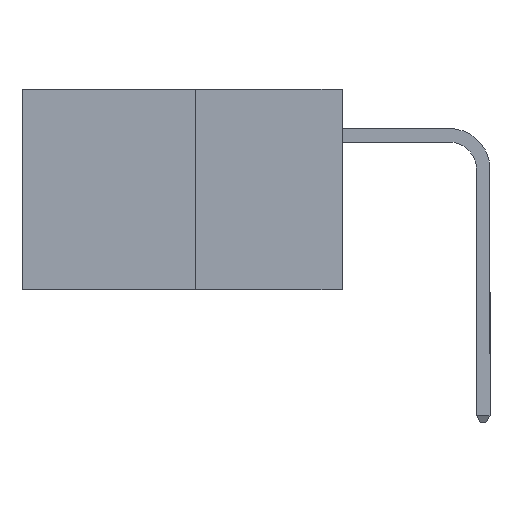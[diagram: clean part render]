
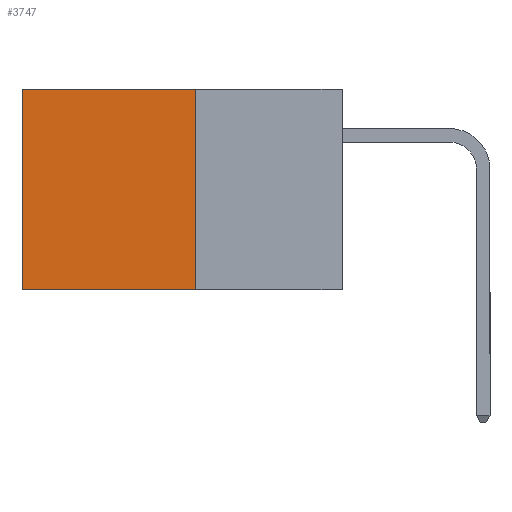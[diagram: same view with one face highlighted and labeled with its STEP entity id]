
A CAD part, left-side view. The second image highlights one B-rep face of the part: STEP entity #3747.
In plain terms, the highlighted planar face has unit normal (-1, 0, 0).
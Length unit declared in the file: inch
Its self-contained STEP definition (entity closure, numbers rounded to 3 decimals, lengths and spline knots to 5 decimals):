
#99 = LINE ( 'NONE', #5122, #6754 ) ;
#448 = DIRECTION ( 'NONE',  ( 0., 0., -1. ) ) ;
#484 = LINE ( 'NONE', #10018, #7142 ) ;
#1225 = ORIENTED_EDGE ( 'NONE', *, *, #4623, .T. ) ;
#1932 = CARTESIAN_POINT ( 'NONE',  ( 0.277, 0.27, -0.37 ) ) ;
#1987 = VECTOR ( 'NONE', #2751, 39.37008 ) ;
#2191 = FACE_OUTER_BOUND ( 'NONE', #2193, .T. ) ;
#2193 = EDGE_LOOP ( 'NONE', ( #1225, #6839, #4777, #4399 ) ) ;
#2557 = CARTESIAN_POINT ( 'NONE',  ( 0.277, 0.27, 0. ) ) ;
#2565 = CARTESIAN_POINT ( 'NONE',  ( 0.277, 0.27, 0. ) ) ;
#2669 = DIRECTION ( 'NONE',  ( 0., 0., -1. ) ) ;
#2751 = DIRECTION ( 'NONE',  ( 0., 1., 0. ) ) ;
#3038 = AXIS2_PLACEMENT_3D ( 'NONE', #4047, #7162, #8775 ) ;
#3365 = DIRECTION ( 'NONE',  ( 0., 1., 0. ) ) ;
#3367 = VECTOR ( 'NONE', #3365, 39.37008 ) ;
#3747 = ADVANCED_FACE ( 'NONE', ( #2191 ), #9639, .F. ) ;
#3955 = CARTESIAN_POINT ( 'NONE',  ( 0.277, 0.59, 0. ) ) ;
#4047 = CARTESIAN_POINT ( 'NONE',  ( 0.277, 0.27, -0.37 ) ) ;
#4272 = VERTEX_POINT ( 'NONE', #3955 ) ;
#4399 = ORIENTED_EDGE ( 'NONE', *, *, #5167, .T. ) ;
#4623 = EDGE_CURVE ( 'NONE', #4272, #8863, #99, .T. ) ;
#4777 = ORIENTED_EDGE ( 'NONE', *, *, #8181, .F. ) ;
#5122 = CARTESIAN_POINT ( 'NONE',  ( 0.277, 0.59, -0.37 ) ) ;
#5167 = EDGE_CURVE ( 'NONE', #7390, #4272, #9720, .T. ) ;
#6754 = VECTOR ( 'NONE', #2669, 39.37008 ) ;
#6839 = ORIENTED_EDGE ( 'NONE', *, *, #8855, .F. ) ;
#7142 = VECTOR ( 'NONE', #448, 39.37008 ) ;
#7162 = DIRECTION ( 'NONE',  ( 1., 0., 0. ) ) ;
#7390 = VERTEX_POINT ( 'NONE', #2565 ) ;
#7517 = CARTESIAN_POINT ( 'NONE',  ( 0.277, 0.59, -0.37 ) ) ;
#8181 = EDGE_CURVE ( 'NONE', #7390, #10346, #484, .T. ) ;
#8357 = LINE ( 'NONE', #1932, #1987 ) ;
#8775 = DIRECTION ( 'NONE',  ( 0., 0., -1. ) ) ;
#8855 = EDGE_CURVE ( 'NONE', #10346, #8863, #8357, .T. ) ;
#8863 = VERTEX_POINT ( 'NONE', #7517 ) ;
#9639 = PLANE ( 'NONE',  #3038 ) ;
#9720 = LINE ( 'NONE', #2557, #3367 ) ;
#10018 = CARTESIAN_POINT ( 'NONE',  ( 0.277, 0.27, -0.37 ) ) ;
#10085 = CARTESIAN_POINT ( 'NONE',  ( 0.277, 0.27, -0.37 ) ) ;
#10346 = VERTEX_POINT ( 'NONE', #10085 ) ;
